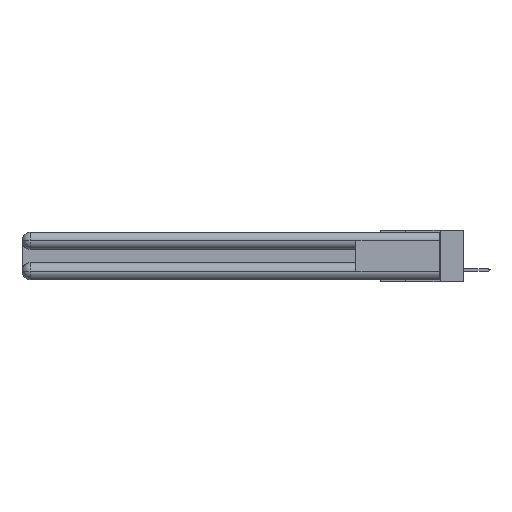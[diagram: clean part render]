
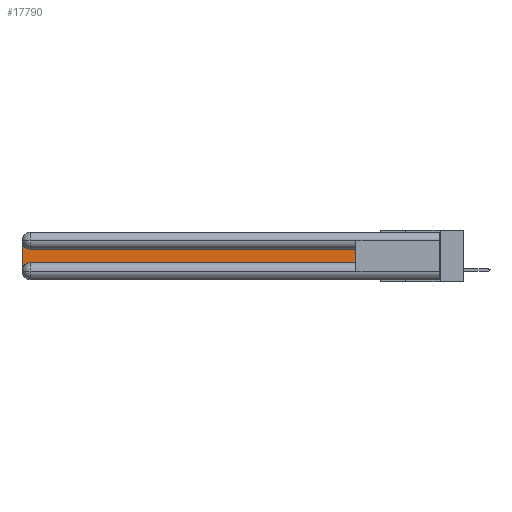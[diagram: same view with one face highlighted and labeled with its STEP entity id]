
A CAD part, left-side view. The second image highlights one B-rep face of the part: STEP entity #17790.
In plain terms, the highlighted planar face has unit normal (-1, 0, 0).
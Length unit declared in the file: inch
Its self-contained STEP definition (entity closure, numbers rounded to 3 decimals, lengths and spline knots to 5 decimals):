
#222 = PLANE ( 'NONE',  #20091 ) ;
#2018 = CARTESIAN_POINT ( 'NONE',  ( 0.075, 0.6, -0.1225 ) ) ;
#2033 = CARTESIAN_POINT ( 'NONE',  ( 0.075, 2.94, -0.1225 ) ) ;
#4052 = DIRECTION ( 'NONE',  ( 0., 1., 0. ) ) ;
#5339 = VECTOR ( 'NONE', #4052, 39.37008 ) ;
#5793 = FACE_OUTER_BOUND ( 'NONE', #28809, .T. ) ;
#5888 = EDGE_CURVE ( 'NONE', #11578, #6850, #13954, .T. ) ;
#6697 = VECTOR ( 'NONE', #16526, 39.37008 ) ;
#6850 = VERTEX_POINT ( 'NONE', #2033 ) ;
#7137 = CARTESIAN_POINT ( 'NONE',  ( 0.075, 3., -0.1225 ) ) ;
#7939 = LINE ( 'NONE', #10359, #12969 ) ;
#8558 = VERTEX_POINT ( 'NONE', #28186 ) ;
#8793 = VERTEX_POINT ( 'NONE', #21018 ) ;
#9578 = LINE ( 'NONE', #23374, #6697 ) ;
#10359 = CARTESIAN_POINT ( 'NONE',  ( 0.075, 3., -0.2175 ) ) ;
#11578 = VERTEX_POINT ( 'NONE', #27121 ) ;
#11707 = AXIS2_PLACEMENT_3D ( 'NONE', #16219, #27965, #11792 ) ;
#11792 = DIRECTION ( 'NONE',  ( 0., 0., -1. ) ) ;
#11813 = EDGE_CURVE ( 'NONE', #19321, #12078, #9578, .T. ) ;
#12078 = VERTEX_POINT ( 'NONE', #24683 ) ;
#12631 = VECTOR ( 'NONE', #26787, 39.37008 ) ;
#12844 = ORIENTED_EDGE ( 'NONE', *, *, #24358, .T. ) ;
#12969 = VECTOR ( 'NONE', #28952, 39.37008 ) ;
#13106 = ORIENTED_EDGE ( 'NONE', *, *, #28837, .T. ) ;
#13243 = ORIENTED_EDGE ( 'NONE', *, *, #15677, .T. ) ;
#13419 = ORIENTED_EDGE ( 'NONE', *, *, #11813, .T. ) ;
#13515 = CIRCLE ( 'NONE', #11707, 0.06 ) ;
#13954 = LINE ( 'NONE', #2018, #5339 ) ;
#14938 = EDGE_CURVE ( 'NONE', #8558, #19321, #17018, .T. ) ;
#15106 = LINE ( 'NONE', #29087, #12631 ) ;
#15677 = EDGE_CURVE ( 'NONE', #8793, #8558, #7939, .T. ) ;
#16219 = CARTESIAN_POINT ( 'NONE',  ( 0.075, 2.94, -0.0625 ) ) ;
#16323 = DIRECTION ( 'NONE',  ( 1., 0., 0. ) ) ;
#16526 = DIRECTION ( 'NONE',  ( 0., -1., 0. ) ) ;
#16615 = DIRECTION ( 'NONE',  ( 1., 0., 0. ) ) ;
#16814 = DIRECTION ( 'NONE',  ( 0., 0., -1. ) ) ;
#17018 = CIRCLE ( 'NONE', #24841, 0.06 ) ;
#17790 = ADVANCED_FACE ( 'NONE', ( #5793 ), #222, .F. ) ;
#19234 = CARTESIAN_POINT ( 'NONE',  ( 0.075, 2.94, -0.2775 ) ) ;
#19321 = VERTEX_POINT ( 'NONE', #28386 ) ;
#19382 = ORIENTED_EDGE ( 'NONE', *, *, #5888, .T. ) ;
#20091 = AXIS2_PLACEMENT_3D ( 'NONE', #7137, #16323, #23260 ) ;
#21018 = CARTESIAN_POINT ( 'NONE',  ( 0.075, 3., -0.0625 ) ) ;
#23260 = DIRECTION ( 'NONE',  ( 0., 0., -1. ) ) ;
#23374 = CARTESIAN_POINT ( 'NONE',  ( 0.075, 0.6, -0.2175 ) ) ;
#24358 = EDGE_CURVE ( 'NONE', #12078, #11578, #15106, .T. ) ;
#24683 = CARTESIAN_POINT ( 'NONE',  ( 0.075, 0.6, -0.2175 ) ) ;
#24841 = AXIS2_PLACEMENT_3D ( 'NONE', #19234, #16615, #16814 ) ;
#26787 = DIRECTION ( 'NONE',  ( 0., 0., 1. ) ) ;
#27121 = CARTESIAN_POINT ( 'NONE',  ( 0.075, 0.6, -0.1225 ) ) ;
#27965 = DIRECTION ( 'NONE',  ( 1., 0., 0. ) ) ;
#28111 = ORIENTED_EDGE ( 'NONE', *, *, #14938, .T. ) ;
#28186 = CARTESIAN_POINT ( 'NONE',  ( 0.075, 3., -0.2775 ) ) ;
#28386 = CARTESIAN_POINT ( 'NONE',  ( 0.075, 2.94, -0.2175 ) ) ;
#28809 = EDGE_LOOP ( 'NONE', ( #19382, #13106, #13243, #28111, #13419, #12844 ) ) ;
#28837 = EDGE_CURVE ( 'NONE', #6850, #8793, #13515, .T. ) ;
#28952 = DIRECTION ( 'NONE',  ( 0., 0., -1. ) ) ;
#29087 = CARTESIAN_POINT ( 'NONE',  ( 0.075, 0.6, -0.2175 ) ) ;
